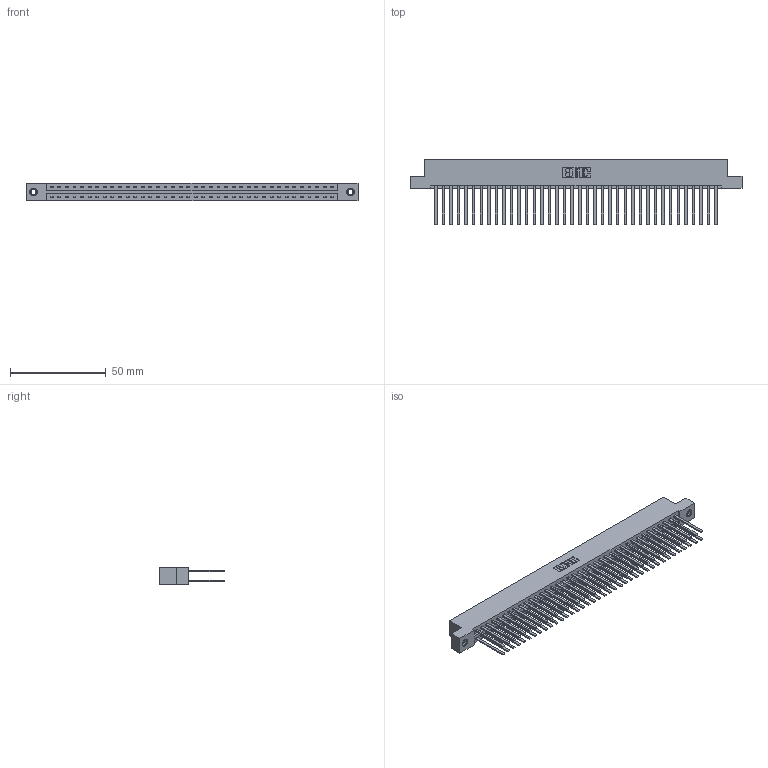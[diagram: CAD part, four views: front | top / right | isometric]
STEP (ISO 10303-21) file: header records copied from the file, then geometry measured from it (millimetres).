
FILE_DESCRIPTION (( 'STEP AP203' ), '1' );
FILE_NAME ('387-076-544-207.STEP', '2018-09-23T15:54:36', ( '' ), ( '' ), 'SwSTEP 2.0', 'SolidWorks 2016', '' );
FILE_SCHEMA (( 'CONFIG_CONTROL_DESIGN' ));
Length unit declared in the file: inch
Products named in the file (4): 345-292-001_345-293-144; 345-250-001_345-250-005-103; 387-076-544-207; 337 Part_Flush Mounting Lugs - 0.156 Dia-TI
Assembly tree (79 placements, depth 2):
  387-076-544-207
    337 Part_Flush Mounting Lugs - 0.156 Dia-TI
    345-292-001_345-293-144  x76
    345-250-001_345-250-005-103  x2
Bounding box: 173.58 x 34.3 x 9.4 mm (x, y, z)
Volume: 19292.2 mm3; surface area: 25287.3 mm2
Topology: 79 solids, 79 shells, 3822 faces, 11315 edges, 7434 vertices
Faces by surface type: plane 2686, cylinder 1120, cone 12, torus 4
Entity records: 30982 total; most frequent: CARTESIAN_POINT 5201, ORIENTED_EDGE 5130, DIRECTION 4459, EDGE_CURVE 2565, VECTOR 2421, LINE 2421, VERTEX_POINT 1704, AXIS2_PLACEMENT_3D 1019
